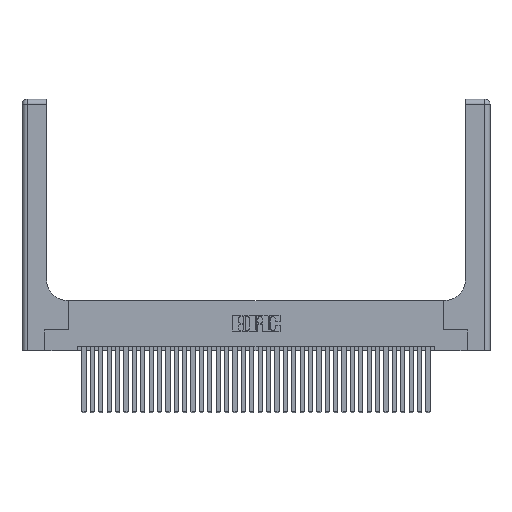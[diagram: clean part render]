
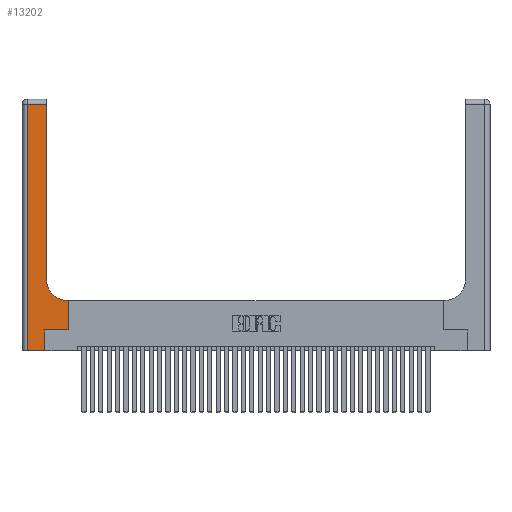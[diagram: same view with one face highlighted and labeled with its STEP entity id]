
A CAD part, top view. The second image highlights one B-rep face of the part: STEP entity #13202.
In plain terms, the highlighted planar face has unit normal (0, 0, 1).
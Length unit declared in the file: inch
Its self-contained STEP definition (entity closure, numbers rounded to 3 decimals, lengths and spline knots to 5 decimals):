
#229 = VERTEX_POINT ( 'NONE', #11185 ) ;
#841 = CARTESIAN_POINT ( 'NONE',  ( 0., 2.94, 0.37 ) ) ;
#1258 = VERTEX_POINT ( 'NONE', #14493 ) ;
#1420 = DIRECTION ( 'NONE',  ( 0., -1., 0. ) ) ;
#1982 = EDGE_CURVE ( 'NONE', #1258, #33727, #37052, .T. ) ;
#2193 = VECTOR ( 'NONE', #35131, 39.37008 ) ;
#2968 = CIRCLE ( 'NONE', #27316, 0.25 ) ;
#3080 = VERTEX_POINT ( 'NONE', #36767 ) ;
#3380 = LINE ( 'NONE', #33433, #33545 ) ;
#3582 = CARTESIAN_POINT ( 'NONE',  ( 0.5415, 0.85, 0.37 ) ) ;
#3693 = EDGE_CURVE ( 'NONE', #15780, #3080, #2968, .T. ) ;
#3944 = CARTESIAN_POINT ( 'NONE',  ( 0.2915, 0.6, 0.37 ) ) ;
#4034 = VECTOR ( 'NONE', #12353, 39.37008 ) ;
#5227 = ORIENTED_EDGE ( 'NONE', *, *, #21398, .T. ) ;
#6223 = VECTOR ( 'NONE', #28324, 39.37008 ) ;
#6478 = LINE ( 'NONE', #18943, #11018 ) ;
#7258 = DIRECTION ( 'NONE',  ( 0., 0., -1. ) ) ;
#7432 = CARTESIAN_POINT ( 'NONE',  ( 0.2915, 2.94, 0.37 ) ) ;
#7668 = CARTESIAN_POINT ( 'NONE',  ( 0.5585, 0.25, 0.37 ) ) ;
#8525 = VERTEX_POINT ( 'NONE', #7432 ) ;
#8978 = DIRECTION ( 'NONE',  ( 0., 1., 0. ) ) ;
#9196 = ORIENTED_EDGE ( 'NONE', *, *, #30187, .T. ) ;
#9782 = ORIENTED_EDGE ( 'NONE', *, *, #19791, .T. ) ;
#10891 = LINE ( 'NONE', #3944, #4034 ) ;
#11018 = VECTOR ( 'NONE', #1420, 39.37008 ) ;
#11185 = CARTESIAN_POINT ( 'NONE',  ( 0.06, 2.94, 0.37 ) ) ;
#12353 = DIRECTION ( 'NONE',  ( -1., 0., 0. ) ) ;
#13024 = VECTOR ( 'NONE', #8978, 39.37008 ) ;
#13202 = ADVANCED_FACE ( 'NONE', ( #32008 ), #23289, .F. ) ;
#13434 = EDGE_CURVE ( 'NONE', #19727, #1258, #36086, .T. ) ;
#14416 = AXIS2_PLACEMENT_3D ( 'NONE', #23534, #17263, #23409 ) ;
#14493 = CARTESIAN_POINT ( 'NONE',  ( 0.5585, 0.25, 0.37 ) ) ;
#15684 = ORIENTED_EDGE ( 'NONE', *, *, #30161, .T. ) ;
#15780 = VERTEX_POINT ( 'NONE', #18276 ) ;
#17263 = DIRECTION ( 'NONE',  ( 0., 0., -1. ) ) ;
#17729 = CARTESIAN_POINT ( 'NONE',  ( 0.269, 0.25, 0.37 ) ) ;
#18276 = CARTESIAN_POINT ( 'NONE',  ( 0.5415, 0.6, 0.37 ) ) ;
#18943 = CARTESIAN_POINT ( 'NONE',  ( 0.06, 3., 0.37 ) ) ;
#18993 = LINE ( 'NONE', #31653, #6223 ) ;
#19727 = VERTEX_POINT ( 'NONE', #24415 ) ;
#19791 = EDGE_CURVE ( 'NONE', #26886, #19727, #28170, .T. ) ;
#21398 = EDGE_CURVE ( 'NONE', #33552, #26886, #3380, .T. ) ;
#21496 = CARTESIAN_POINT ( 'NONE',  ( 0.269, 0., 0.37 ) ) ;
#22011 = CARTESIAN_POINT ( 'NONE',  ( 0.06, 0., 0.37 ) ) ;
#23289 = PLANE ( 'NONE',  #14416 ) ;
#23409 = DIRECTION ( 'NONE',  ( -1., 0., 0. ) ) ;
#23534 = CARTESIAN_POINT ( 'NONE',  ( 0., 3., 0.37 ) ) ;
#24293 = DIRECTION ( 'NONE',  ( -1., 0., 0. ) ) ;
#24415 = CARTESIAN_POINT ( 'NONE',  ( 0.269, 0.25, 0.37 ) ) ;
#24953 = EDGE_CURVE ( 'NONE', #229, #33552, #6478, .T. ) ;
#26568 = CARTESIAN_POINT ( 'NONE',  ( 0.5585, 0.6, 0.37 ) ) ;
#26794 = ORIENTED_EDGE ( 'NONE', *, *, #13434, .T. ) ;
#26886 = VERTEX_POINT ( 'NONE', #21496 ) ;
#26906 = ORIENTED_EDGE ( 'NONE', *, *, #3693, .T. ) ;
#27316 = AXIS2_PLACEMENT_3D ( 'NONE', #3582, #7258, #36734 ) ;
#27412 = EDGE_LOOP ( 'NONE', ( #35495, #15684, #31030, #5227, #9782, #26794, #36437, #9196, #26906 ) ) ;
#28170 = LINE ( 'NONE', #34226, #13024 ) ;
#28324 = DIRECTION ( 'NONE',  ( 0., 1., 0. ) ) ;
#30161 = EDGE_CURVE ( 'NONE', #8525, #229, #36108, .T. ) ;
#30187 = EDGE_CURVE ( 'NONE', #33727, #15780, #10891, .T. ) ;
#30559 = VECTOR ( 'NONE', #24293, 39.37008 ) ;
#30604 = DIRECTION ( 'NONE',  ( 1., 0., 0. ) ) ;
#31030 = ORIENTED_EDGE ( 'NONE', *, *, #24953, .T. ) ;
#31653 = CARTESIAN_POINT ( 'NONE',  ( 0.2915, 3., 0.37 ) ) ;
#32008 = FACE_OUTER_BOUND ( 'NONE', #27412, .T. ) ;
#32494 = EDGE_CURVE ( 'NONE', #3080, #8525, #18993, .T. ) ;
#33433 = CARTESIAN_POINT ( 'NONE',  ( 0., 0., 0.37 ) ) ;
#33545 = VECTOR ( 'NONE', #30604, 39.37008 ) ;
#33552 = VERTEX_POINT ( 'NONE', #22011 ) ;
#33727 = VERTEX_POINT ( 'NONE', #26568 ) ;
#33779 = DIRECTION ( 'NONE',  ( 0., 1., 0. ) ) ;
#34226 = CARTESIAN_POINT ( 'NONE',  ( 0.269, 0., 0.37 ) ) ;
#35131 = DIRECTION ( 'NONE',  ( 1., 0., 0. ) ) ;
#35495 = ORIENTED_EDGE ( 'NONE', *, *, #32494, .T. ) ;
#36086 = LINE ( 'NONE', #17729, #2193 ) ;
#36108 = LINE ( 'NONE', #841, #30559 ) ;
#36437 = ORIENTED_EDGE ( 'NONE', *, *, #1982, .T. ) ;
#36734 = DIRECTION ( 'NONE',  ( 1., 0., 0. ) ) ;
#36767 = CARTESIAN_POINT ( 'NONE',  ( 0.2915, 0.85, 0.37 ) ) ;
#37052 = LINE ( 'NONE', #7668, #37506 ) ;
#37506 = VECTOR ( 'NONE', #33779, 39.37008 ) ;
